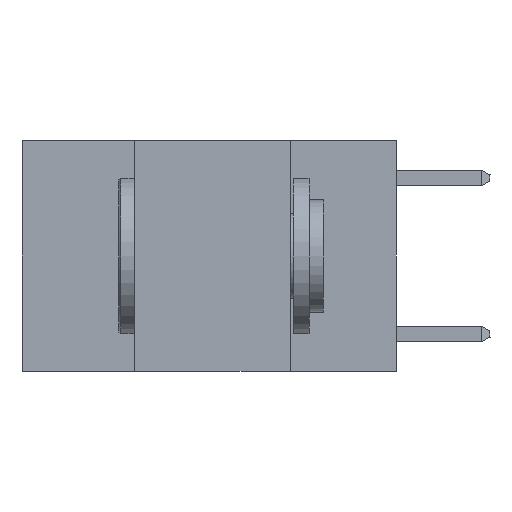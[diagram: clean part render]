
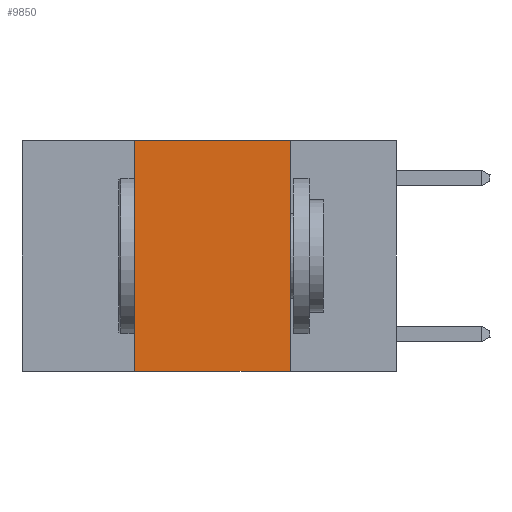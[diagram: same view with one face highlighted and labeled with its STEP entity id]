
A CAD part, left-side view. The second image highlights one B-rep face of the part: STEP entity #9850.
In plain terms, the highlighted planar face has unit normal (-1, 0, 0).
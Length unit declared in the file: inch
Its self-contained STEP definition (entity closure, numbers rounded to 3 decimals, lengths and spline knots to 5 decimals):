
#812 = VERTEX_POINT ( 'NONE', #13949 ) ;
#1024 = VERTEX_POINT ( 'NONE', #14420 ) ;
#1493 = EDGE_CURVE ( 'NONE', #812, #1024, #15675, .T. ) ;
#1768 = VERTEX_POINT ( 'NONE', #6624 ) ;
#1941 = LINE ( 'NONE', #5571, #12297 ) ;
#2040 = ORIENTED_EDGE ( 'NONE', *, *, #12409, .T. ) ;
#2533 = DIRECTION ( 'NONE',  ( 0., 0., 1. ) ) ;
#3140 = VECTOR ( 'NONE', #2533, 39.37008 ) ;
#3336 = VECTOR ( 'NONE', #6505, 39.37008 ) ;
#3811 = PLANE ( 'NONE',  #4076 ) ;
#3887 = FACE_OUTER_BOUND ( 'NONE', #14171, .T. ) ;
#4076 = AXIS2_PLACEMENT_3D ( 'NONE', #7594, #10073, #5114 ) ;
#5113 = LINE ( 'NONE', #7660, #3140 ) ;
#5114 = DIRECTION ( 'NONE',  ( 0., 0., -1. ) ) ;
#5225 = LINE ( 'NONE', #10101, #3336 ) ;
#5571 = CARTESIAN_POINT ( 'NONE',  ( 0., 0.6, -0.37 ) ) ;
#6224 = DIRECTION ( 'NONE',  ( 0., 0., -1. ) ) ;
#6505 = DIRECTION ( 'NONE',  ( 0., -1., 0. ) ) ;
#6624 = CARTESIAN_POINT ( 'NONE',  ( 0., 0.42, -0.37 ) ) ;
#7263 = CARTESIAN_POINT ( 'NONE',  ( 0., 0.17, 0. ) ) ;
#7358 = ORIENTED_EDGE ( 'NONE', *, *, #13169, .F. ) ;
#7594 = CARTESIAN_POINT ( 'NONE',  ( 0., 0.6, 0. ) ) ;
#7660 = CARTESIAN_POINT ( 'NONE',  ( 0., 0.42, 0. ) ) ;
#9850 = ADVANCED_FACE ( 'NONE', ( #3887 ), #3811, .F. ) ;
#10073 = DIRECTION ( 'NONE',  ( 1., 0., 0. ) ) ;
#10101 = CARTESIAN_POINT ( 'NONE',  ( 0., 0.6, 0. ) ) ;
#10172 = VERTEX_POINT ( 'NONE', #11936 ) ;
#11936 = CARTESIAN_POINT ( 'NONE',  ( 0., 0.42, 0. ) ) ;
#12297 = VECTOR ( 'NONE', #15399, 39.37008 ) ;
#12409 = EDGE_CURVE ( 'NONE', #1768, #1024, #1941, .T. ) ;
#12642 = ORIENTED_EDGE ( 'NONE', *, *, #1493, .F. ) ;
#12954 = ORIENTED_EDGE ( 'NONE', *, *, #15502, .F. ) ;
#13169 = EDGE_CURVE ( 'NONE', #10172, #812, #5225, .T. ) ;
#13919 = VECTOR ( 'NONE', #6224, 39.37008 ) ;
#13949 = CARTESIAN_POINT ( 'NONE',  ( 0., 0.17, 0. ) ) ;
#14171 = EDGE_LOOP ( 'NONE', ( #12642, #7358, #12954, #2040 ) ) ;
#14420 = CARTESIAN_POINT ( 'NONE',  ( 0., 0.17, -0.37 ) ) ;
#15399 = DIRECTION ( 'NONE',  ( 0., -1., 0. ) ) ;
#15502 = EDGE_CURVE ( 'NONE', #1768, #10172, #5113, .T. ) ;
#15675 = LINE ( 'NONE', #7263, #13919 ) ;
